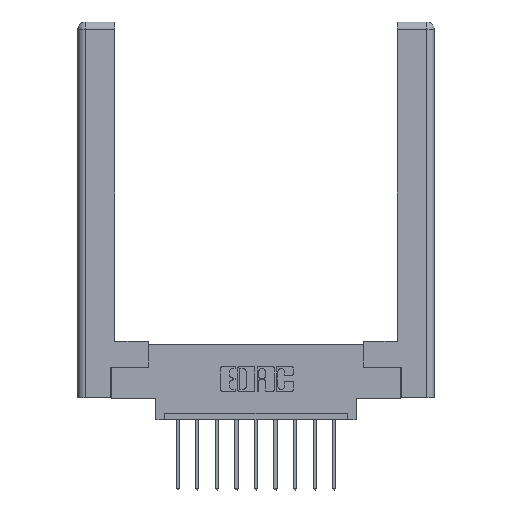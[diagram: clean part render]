
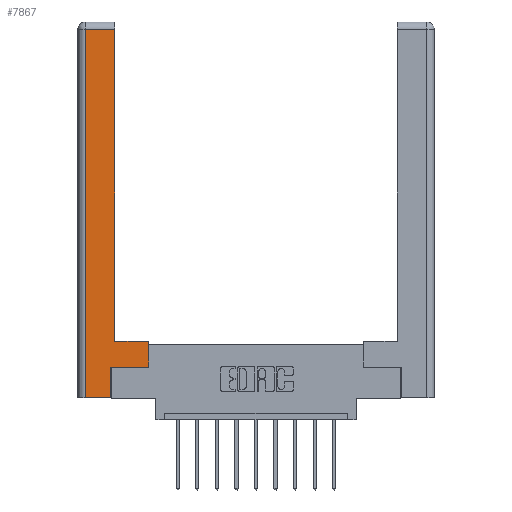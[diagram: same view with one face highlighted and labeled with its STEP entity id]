
A CAD part, top view. The second image highlights one B-rep face of the part: STEP entity #7867.
In plain terms, the highlighted planar face has unit normal (0, 0, 1).
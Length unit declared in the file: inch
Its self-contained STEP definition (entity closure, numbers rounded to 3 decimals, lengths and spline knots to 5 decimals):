
#226 = PLANE ( 'NONE',  #8870 ) ;
#450 = CARTESIAN_POINT ( 'NONE',  ( 0.565, 0.45, 0. ) ) ;
#472 = ORIENTED_EDGE ( 'NONE', *, *, #4190, .T. ) ;
#746 = VERTEX_POINT ( 'NONE', #1050 ) ;
#1050 = CARTESIAN_POINT ( 'NONE',  ( 0.295, 0.45, 0. ) ) ;
#1081 = ORIENTED_EDGE ( 'NONE', *, *, #5231, .T. ) ;
#1537 = ORIENTED_EDGE ( 'NONE', *, *, #10703, .T. ) ;
#1571 = CARTESIAN_POINT ( 'NONE',  ( 0.0615, 0., 0. ) ) ;
#1660 = ORIENTED_EDGE ( 'NONE', *, *, #3384, .T. ) ;
#1666 = EDGE_LOOP ( 'NONE', ( #6182, #10475, #1660, #6305, #1537, #2895, #472, #1081 ) ) ;
#1716 = EDGE_CURVE ( 'NONE', #10496, #3915, #7101, .T. ) ;
#2414 = VECTOR ( 'NONE', #5730, 39.37008 ) ;
#2454 = VECTOR ( 'NONE', #6542, 39.37008 ) ;
#2611 = CARTESIAN_POINT ( 'NONE',  ( 0.0615, 2.94, 0. ) ) ;
#2620 = DIRECTION ( 'NONE',  ( 0., -1., 0. ) ) ;
#2834 = CARTESIAN_POINT ( 'NONE',  ( 0.295, 0.45, 0. ) ) ;
#2895 = ORIENTED_EDGE ( 'NONE', *, *, #4866, .T. ) ;
#2901 = LINE ( 'NONE', #2834, #13546 ) ;
#3384 = EDGE_CURVE ( 'NONE', #11262, #10496, #9471, .T. ) ;
#3438 = CARTESIAN_POINT ( 'NONE',  ( 0.265, 0.245, 0. ) ) ;
#3602 = LINE ( 'NONE', #450, #9287 ) ;
#3907 = DIRECTION ( 'NONE',  ( -1., 0., 0. ) ) ;
#3915 = VERTEX_POINT ( 'NONE', #11776 ) ;
#4190 = EDGE_CURVE ( 'NONE', #12303, #7040, #3602, .T. ) ;
#4210 = CARTESIAN_POINT ( 'NONE',  ( 0.295, 3., 0. ) ) ;
#4672 = CARTESIAN_POINT ( 'NONE',  ( 0.265, 0., 0. ) ) ;
#4866 = EDGE_CURVE ( 'NONE', #8359, #12303, #7580, .T. ) ;
#5231 = EDGE_CURVE ( 'NONE', #7040, #746, #2901, .T. ) ;
#5288 = CARTESIAN_POINT ( 'NONE',  ( 0.295, 2.94, 0. ) ) ;
#5707 = EDGE_CURVE ( 'NONE', #11322, #11262, #8054, .T. ) ;
#5730 = DIRECTION ( 'NONE',  ( -1., 0., 0. ) ) ;
#6182 = ORIENTED_EDGE ( 'NONE', *, *, #8958, .T. ) ;
#6305 = ORIENTED_EDGE ( 'NONE', *, *, #1716, .T. ) ;
#6502 = CARTESIAN_POINT ( 'NONE',  ( 0.565, 0.245, 0. ) ) ;
#6542 = DIRECTION ( 'NONE',  ( 0., 1., 0. ) ) ;
#6955 = DIRECTION ( 'NONE',  ( 1., 0., 0. ) ) ;
#7040 = VERTEX_POINT ( 'NONE', #7238 ) ;
#7101 = LINE ( 'NONE', #4672, #12561 ) ;
#7238 = CARTESIAN_POINT ( 'NONE',  ( 0.565, 0.45, 0. ) ) ;
#7580 = LINE ( 'NONE', #6502, #7920 ) ;
#7803 = VECTOR ( 'NONE', #2620, 39.37008 ) ;
#7806 = CARTESIAN_POINT ( 'NONE',  ( 0., 0., 0. ) ) ;
#7867 = ADVANCED_FACE ( 'NONE', ( #13306 ), #226, .F. ) ;
#7920 = VECTOR ( 'NONE', #8626, 39.37008 ) ;
#8054 = LINE ( 'NONE', #2611, #2414 ) ;
#8359 = VERTEX_POINT ( 'NONE', #8643 ) ;
#8626 = DIRECTION ( 'NONE',  ( 1., 0., 0. ) ) ;
#8643 = CARTESIAN_POINT ( 'NONE',  ( 0.265, 0.245, 0. ) ) ;
#8870 = AXIS2_PLACEMENT_3D ( 'NONE', #7806, #8883, #9946 ) ;
#8883 = DIRECTION ( 'NONE',  ( 0., 0., -1. ) ) ;
#8958 = EDGE_CURVE ( 'NONE', #746, #11322, #9658, .T. ) ;
#9287 = VECTOR ( 'NONE', #13235, 39.37008 ) ;
#9326 = CARTESIAN_POINT ( 'NONE',  ( 0.565, 0.245, 0. ) ) ;
#9471 = LINE ( 'NONE', #13250, #7803 ) ;
#9658 = LINE ( 'NONE', #4210, #10636 ) ;
#9946 = DIRECTION ( 'NONE',  ( -1., 0., 0. ) ) ;
#10475 = ORIENTED_EDGE ( 'NONE', *, *, #5707, .T. ) ;
#10496 = VERTEX_POINT ( 'NONE', #1571 ) ;
#10636 = VECTOR ( 'NONE', #11657, 39.37008 ) ;
#10703 = EDGE_CURVE ( 'NONE', #3915, #8359, #10938, .T. ) ;
#10938 = LINE ( 'NONE', #3438, #2454 ) ;
#11262 = VERTEX_POINT ( 'NONE', #12060 ) ;
#11322 = VERTEX_POINT ( 'NONE', #5288 ) ;
#11657 = DIRECTION ( 'NONE',  ( 0., 1., 0. ) ) ;
#11776 = CARTESIAN_POINT ( 'NONE',  ( 0.265, 0., 0. ) ) ;
#12060 = CARTESIAN_POINT ( 'NONE',  ( 0.0615, 2.94, 0. ) ) ;
#12303 = VERTEX_POINT ( 'NONE', #9326 ) ;
#12561 = VECTOR ( 'NONE', #6955, 39.37008 ) ;
#13235 = DIRECTION ( 'NONE',  ( 0., 1., 0. ) ) ;
#13250 = CARTESIAN_POINT ( 'NONE',  ( 0.0615, 0., 0. ) ) ;
#13306 = FACE_OUTER_BOUND ( 'NONE', #1666, .T. ) ;
#13546 = VECTOR ( 'NONE', #3907, 39.37008 ) ;
